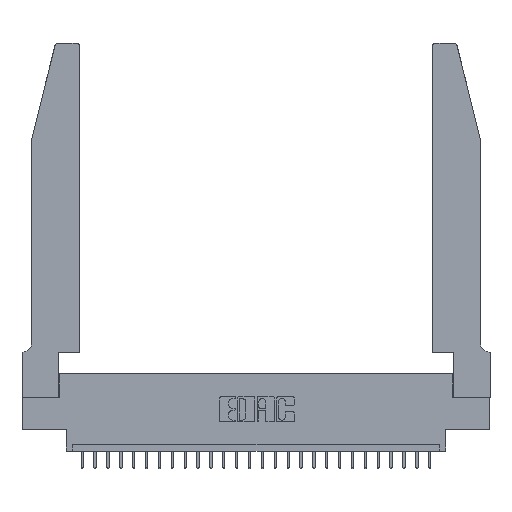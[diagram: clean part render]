
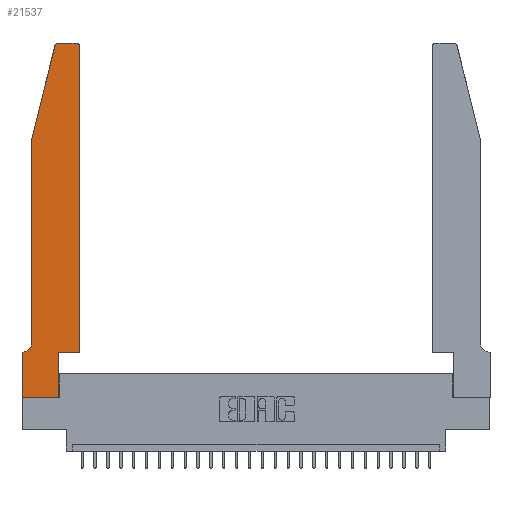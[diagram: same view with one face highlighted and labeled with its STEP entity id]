
A CAD part, top view. The second image highlights one B-rep face of the part: STEP entity #21537.
In plain terms, the highlighted planar face has unit normal (0, 0, 1).
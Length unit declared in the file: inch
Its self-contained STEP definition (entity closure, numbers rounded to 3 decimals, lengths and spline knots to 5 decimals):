
#149 = EDGE_CURVE ( 'NONE', #5961, #4030, #20637, .T. ) ;
#580 = VECTOR ( 'NONE', #24339, 39.37008 ) ;
#803 = CARTESIAN_POINT ( 'NONE',  ( 0.4205, 2.75, 0.37 ) ) ;
#1333 = DIRECTION ( 'NONE',  ( 1., 0., 0. ) ) ;
#1549 = CARTESIAN_POINT ( 'NONE',  ( 0., 0.35, 0.37 ) ) ;
#1916 = EDGE_CURVE ( 'NONE', #5978, #3180, #6329, .T. ) ;
#2098 = DIRECTION ( 'NONE',  ( 0., -1., 0. ) ) ;
#3020 = DIRECTION ( 'NONE',  ( 0., 0., -1. ) ) ;
#3064 = VECTOR ( 'NONE', #6707, 39.37008 ) ;
#3180 = VERTEX_POINT ( 'NONE', #6987 ) ;
#3504 = CARTESIAN_POINT ( 'NONE',  ( 0., 0.35, 0.37 ) ) ;
#3659 = DIRECTION ( 'NONE',  ( 1., 0., 0. ) ) ;
#4030 = VERTEX_POINT ( 'NONE', #18098 ) ;
#4219 = VERTEX_POINT ( 'NONE', #1549 ) ;
#5233 = AXIS2_PLACEMENT_3D ( 'NONE', #13685, #9176, #9443 ) ;
#5412 = VECTOR ( 'NONE', #13369, 39.37008 ) ;
#5866 = CARTESIAN_POINT ( 'NONE',  ( 0.2865, 0., 0.37 ) ) ;
#5961 = VERTEX_POINT ( 'NONE', #26335 ) ;
#5978 = VERTEX_POINT ( 'NONE', #16199 ) ;
#6329 = CIRCLE ( 'NONE', #20252, 0.03 ) ;
#6412 = EDGE_CURVE ( 'NONE', #18875, #24195, #17860, .T. ) ;
#6707 = DIRECTION ( 'NONE',  ( -1., 0., 0. ) ) ;
#6987 = CARTESIAN_POINT ( 'NONE',  ( 0.25487, 2.72718, 0.37 ) ) ;
#7398 = VECTOR ( 'NONE', #8285, 39.37008 ) ;
#7518 = VECTOR ( 'NONE', #22439, 39.37008 ) ;
#7623 = FACE_OUTER_BOUND ( 'NONE', #15169, .T. ) ;
#7944 = EDGE_CURVE ( 'NONE', #20289, #5978, #9153, .T. ) ;
#7986 = VECTOR ( 'NONE', #10537, 39.37008 ) ;
#8155 = ORIENTED_EDGE ( 'NONE', *, *, #8336, .T. ) ;
#8285 = DIRECTION ( 'NONE',  ( 0., -1., 0. ) ) ;
#8336 = EDGE_CURVE ( 'NONE', #4030, #4219, #11373, .T. ) ;
#8798 = ORIENTED_EDGE ( 'NONE', *, *, #23921, .T. ) ;
#9153 = LINE ( 'NONE', #17731, #580 ) ;
#9176 = DIRECTION ( 'NONE',  ( 0., 0., 1. ) ) ;
#9366 = VERTEX_POINT ( 'NONE', #23208 ) ;
#9433 = CARTESIAN_POINT ( 'NONE',  ( 0.2865, 0.35, 0.37 ) ) ;
#9443 = DIRECTION ( 'NONE',  ( 1., 0., 0. ) ) ;
#10537 = DIRECTION ( 'NONE',  ( 0., 1., 0. ) ) ;
#11081 = ORIENTED_EDGE ( 'NONE', *, *, #149, .T. ) ;
#11141 = ORIENTED_EDGE ( 'NONE', *, *, #16528, .T. ) ;
#11197 = DIRECTION ( 'NONE',  ( -0.239, -0.971, 0. ) ) ;
#11198 = AXIS2_PLACEMENT_3D ( 'NONE', #3504, #16090, #3659 ) ;
#11373 = LINE ( 'NONE', #15171, #3064 ) ;
#11880 = CARTESIAN_POINT ( 'NONE',  ( 0., 0., 0.37 ) ) ;
#11886 = CARTESIAN_POINT ( 'NONE',  ( 0.284, 2.72, 0.37 ) ) ;
#11920 = VERTEX_POINT ( 'NONE', #15941 ) ;
#12440 = CARTESIAN_POINT ( 'NONE',  ( 0.4505, 0.35, 0.37 ) ) ;
#12875 = LINE ( 'NONE', #14701, #25315 ) ;
#12963 = ORIENTED_EDGE ( 'NONE', *, *, #1916, .T. ) ;
#13369 = DIRECTION ( 'NONE',  ( 1., 0., 0. ) ) ;
#13494 = EDGE_CURVE ( 'NONE', #4219, #18875, #12875, .T. ) ;
#13685 = CARTESIAN_POINT ( 'NONE',  ( 0.4205, 2.72, 0.37 ) ) ;
#13828 = EDGE_CURVE ( 'NONE', #23614, #19027, #20673, .T. ) ;
#14162 = LINE ( 'NONE', #22734, #7518 ) ;
#14318 = EDGE_CURVE ( 'NONE', #3180, #11920, #17113, .T. ) ;
#14701 = CARTESIAN_POINT ( 'NONE',  ( 0., 0., 0.37 ) ) ;
#15164 = ORIENTED_EDGE ( 'NONE', *, *, #21171, .T. ) ;
#15169 = EDGE_LOOP ( 'NONE', ( #26498, #12963, #23268, #11141, #11081, #8155, #26161, #19791, #8798, #24763, #15164, #17002 ) ) ;
#15171 = CARTESIAN_POINT ( 'NONE',  ( 0.0755, 0.35, 0.37 ) ) ;
#15432 = VECTOR ( 'NONE', #11197, 39.37008 ) ;
#15941 = CARTESIAN_POINT ( 'NONE',  ( 0.0755, 2., 0.37 ) ) ;
#16090 = DIRECTION ( 'NONE',  ( 0., 0., 1. ) ) ;
#16171 = AXIS2_PLACEMENT_3D ( 'NONE', #26586, #3020, #24743 ) ;
#16199 = CARTESIAN_POINT ( 'NONE',  ( 0.284, 2.75, 0.37 ) ) ;
#16460 = CARTESIAN_POINT ( 'NONE',  ( 0.4505, 0.35, 0.37 ) ) ;
#16528 = EDGE_CURVE ( 'NONE', #11920, #5961, #18991, .T. ) ;
#17002 = ORIENTED_EDGE ( 'NONE', *, *, #22956, .T. ) ;
#17009 = LINE ( 'NONE', #17432, #7986 ) ;
#17113 = LINE ( 'NONE', #23458, #15432 ) ;
#17394 = CIRCLE ( 'NONE', #5233, 0.03 ) ;
#17432 = CARTESIAN_POINT ( 'NONE',  ( 0.2865, 0.35, 0.37 ) ) ;
#17731 = CARTESIAN_POINT ( 'NONE',  ( 0.2605, 2.75, 0.37 ) ) ;
#17860 = LINE ( 'NONE', #26439, #5412 ) ;
#18098 = CARTESIAN_POINT ( 'NONE',  ( 0.0055, 0.35, 0.37 ) ) ;
#18327 = PLANE ( 'NONE',  #11198 ) ;
#18875 = VERTEX_POINT ( 'NONE', #11880 ) ;
#18991 = LINE ( 'NONE', #27595, #7398 ) ;
#19027 = VERTEX_POINT ( 'NONE', #12440 ) ;
#19791 = ORIENTED_EDGE ( 'NONE', *, *, #6412, .T. ) ;
#20252 = AXIS2_PLACEMENT_3D ( 'NONE', #11886, #20452, #26374 ) ;
#20289 = VERTEX_POINT ( 'NONE', #803 ) ;
#20452 = DIRECTION ( 'NONE',  ( 0., 0., 1. ) ) ;
#20637 = CIRCLE ( 'NONE', #16171, 0.07 ) ;
#20673 = LINE ( 'NONE', #16460, #27119 ) ;
#21171 = EDGE_CURVE ( 'NONE', #19027, #9366, #14162, .T. ) ;
#21537 = ADVANCED_FACE ( 'NONE', ( #7623 ), #18327, .T. ) ;
#22439 = DIRECTION ( 'NONE',  ( 0., 1., 0. ) ) ;
#22734 = CARTESIAN_POINT ( 'NONE',  ( 0.4505, 0.35, 0.37 ) ) ;
#22956 = EDGE_CURVE ( 'NONE', #9366, #20289, #17394, .T. ) ;
#23208 = CARTESIAN_POINT ( 'NONE',  ( 0.4505, 2.72, 0.37 ) ) ;
#23268 = ORIENTED_EDGE ( 'NONE', *, *, #14318, .T. ) ;
#23458 = CARTESIAN_POINT ( 'NONE',  ( 0.0755, 2., 0.37 ) ) ;
#23614 = VERTEX_POINT ( 'NONE', #9433 ) ;
#23921 = EDGE_CURVE ( 'NONE', #24195, #23614, #17009, .T. ) ;
#24195 = VERTEX_POINT ( 'NONE', #5866 ) ;
#24339 = DIRECTION ( 'NONE',  ( -1., 0., 0. ) ) ;
#24743 = DIRECTION ( 'NONE',  ( -1., 0., 0. ) ) ;
#24763 = ORIENTED_EDGE ( 'NONE', *, *, #13828, .T. ) ;
#25315 = VECTOR ( 'NONE', #2098, 39.37008 ) ;
#26161 = ORIENTED_EDGE ( 'NONE', *, *, #13494, .T. ) ;
#26335 = CARTESIAN_POINT ( 'NONE',  ( 0.0755, 0.42, 0.37 ) ) ;
#26374 = DIRECTION ( 'NONE',  ( 1., 0., 0. ) ) ;
#26439 = CARTESIAN_POINT ( 'NONE',  ( 0., 0., 0.37 ) ) ;
#26498 = ORIENTED_EDGE ( 'NONE', *, *, #7944, .T. ) ;
#26586 = CARTESIAN_POINT ( 'NONE',  ( 0.0055, 0.42, 0.37 ) ) ;
#27119 = VECTOR ( 'NONE', #1333, 39.37008 ) ;
#27595 = CARTESIAN_POINT ( 'NONE',  ( 0.0755, 2., 0.37 ) ) ;
